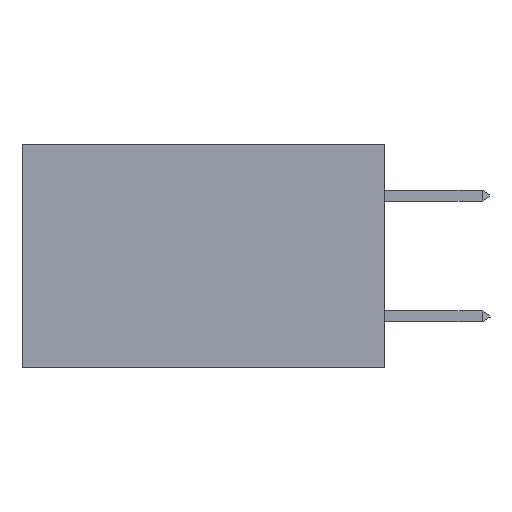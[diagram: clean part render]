
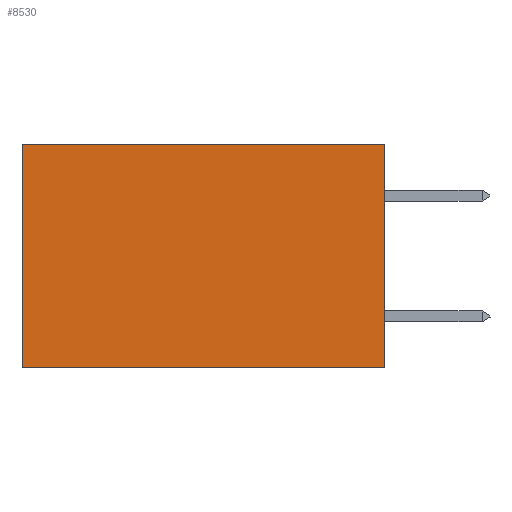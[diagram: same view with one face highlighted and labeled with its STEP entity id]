
A CAD part, left-side view. The second image highlights one B-rep face of the part: STEP entity #8530.
In plain terms, the highlighted planar face has unit normal (-1, 0, 0).
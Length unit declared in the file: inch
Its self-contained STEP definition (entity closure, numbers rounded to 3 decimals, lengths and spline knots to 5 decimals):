
#412 = CARTESIAN_POINT ( 'NONE',  ( 0.2875, 0., -0.37 ) ) ;
#1227 = ORIENTED_EDGE ( 'NONE', *, *, #10738, .T. ) ;
#2447 = CARTESIAN_POINT ( 'NONE',  ( 0.2875, 0., 0. ) ) ;
#4631 = DIRECTION ( 'NONE',  ( 0., 1., 0. ) ) ;
#4817 = LINE ( 'NONE', #24008, #23036 ) ;
#5542 = VERTEX_POINT ( 'NONE', #23591 ) ;
#5739 = VERTEX_POINT ( 'NONE', #23389 ) ;
#7423 = EDGE_CURVE ( 'NONE', #25640, #5542, #25231, .T. ) ;
#8011 = CARTESIAN_POINT ( 'NONE',  ( 0.2875, 0.6, 0. ) ) ;
#8530 = ADVANCED_FACE ( 'NONE', ( #9541 ), #21527, .F. ) ;
#9541 = FACE_OUTER_BOUND ( 'NONE', #17422, .T. ) ;
#10738 = EDGE_CURVE ( 'NONE', #23755, #5542, #18531, .T. ) ;
#11068 = LINE ( 'NONE', #20338, #24433 ) ;
#12913 = ORIENTED_EDGE ( 'NONE', *, *, #7423, .F. ) ;
#13027 = DIRECTION ( 'NONE',  ( 0., 0., -1. ) ) ;
#13228 = AXIS2_PLACEMENT_3D ( 'NONE', #2447, #15214, #13027 ) ;
#13676 = DIRECTION ( 'NONE',  ( 0., 0., -1. ) ) ;
#14558 = CARTESIAN_POINT ( 'NONE',  ( 0.2875, 0., -0.37 ) ) ;
#15214 = DIRECTION ( 'NONE',  ( 1., 0., 0. ) ) ;
#17422 = EDGE_LOOP ( 'NONE', ( #1227, #12913, #26372, #22100 ) ) ;
#18531 = LINE ( 'NONE', #20841, #26650 ) ;
#19187 = EDGE_CURVE ( 'NONE', #5739, #25640, #4817, .T. ) ;
#20338 = CARTESIAN_POINT ( 'NONE',  ( 0.2875, 0., 0. ) ) ;
#20841 = CARTESIAN_POINT ( 'NONE',  ( 0.2875, 0.6, 0. ) ) ;
#21083 = DIRECTION ( 'NONE',  ( 0., 1., 0. ) ) ;
#21527 = PLANE ( 'NONE',  #13228 ) ;
#22100 = ORIENTED_EDGE ( 'NONE', *, *, #23466, .T. ) ;
#23036 = VECTOR ( 'NONE', #13676, 39.37008 ) ;
#23389 = CARTESIAN_POINT ( 'NONE',  ( 0.2875, 0., 0. ) ) ;
#23466 = EDGE_CURVE ( 'NONE', #5739, #23755, #11068, .T. ) ;
#23566 = DIRECTION ( 'NONE',  ( 0., 0., -1. ) ) ;
#23591 = CARTESIAN_POINT ( 'NONE',  ( 0.2875, 0.6, -0.37 ) ) ;
#23755 = VERTEX_POINT ( 'NONE', #8011 ) ;
#24008 = CARTESIAN_POINT ( 'NONE',  ( 0.2875, 0., 0. ) ) ;
#24433 = VECTOR ( 'NONE', #21083, 39.37008 ) ;
#24602 = VECTOR ( 'NONE', #4631, 39.37008 ) ;
#25231 = LINE ( 'NONE', #412, #24602 ) ;
#25640 = VERTEX_POINT ( 'NONE', #14558 ) ;
#26372 = ORIENTED_EDGE ( 'NONE', *, *, #19187, .F. ) ;
#26650 = VECTOR ( 'NONE', #23566, 39.37008 ) ;
